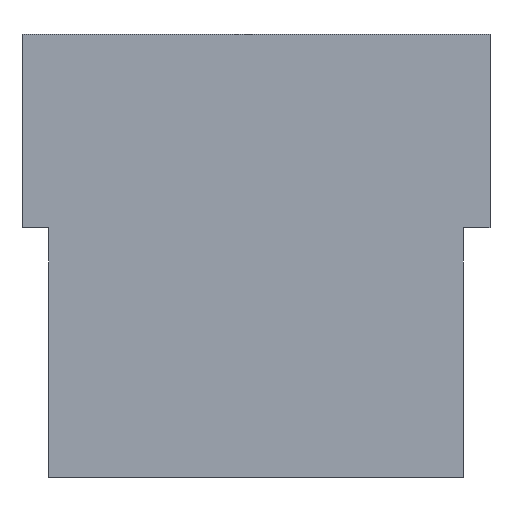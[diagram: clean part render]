
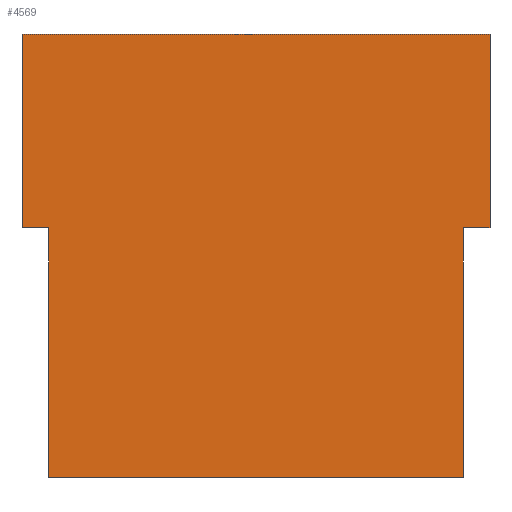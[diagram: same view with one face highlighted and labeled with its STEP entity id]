
A CAD part, front view. The second image highlights one B-rep face of the part: STEP entity #4569.
In plain terms, the highlighted planar face has unit normal (0, -1, 0).
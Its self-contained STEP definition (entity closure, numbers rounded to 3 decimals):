
#89 = VERTEX_POINT ( 'NONE', #2042 ) ;
#93 = EDGE_CURVE ( 'NONE', #89, #4918, #3731, .T. ) ;
#120 = EDGE_CURVE ( 'NONE', #4918, #233, #3376, .T. ) ;
#163 = LINE ( 'NONE', #4018, #1761 ) ;
#189 = CARTESIAN_POINT ( 'NONE',  ( 6.65, -3.15, -7.1 ) ) ;
#223 = DIRECTION ( 'NONE',  ( 0., 1., 0. ) ) ;
#233 = VERTEX_POINT ( 'NONE', #2596 ) ;
#333 = ORIENTED_EDGE ( 'NONE', *, *, #1063, .F. ) ;
#367 = VECTOR ( 'NONE', #423, 1000. ) ;
#370 = CARTESIAN_POINT ( 'NONE',  ( 7.5, -3.15, 0.9 ) ) ;
#423 = DIRECTION ( 'NONE',  ( 1., 0., 0. ) ) ;
#575 = VECTOR ( 'NONE', #2859, 1000. ) ;
#775 = PLANE ( 'NONE',  #2057 ) ;
#853 = ORIENTED_EDGE ( 'NONE', *, *, #120, .F. ) ;
#1063 = EDGE_CURVE ( 'NONE', #4021, #5097, #4996, .T. ) ;
#1168 = CARTESIAN_POINT ( 'NONE',  ( 7.5, -3.15, 7.1 ) ) ;
#1298 = VERTEX_POINT ( 'NONE', #2502 ) ;
#1385 = CARTESIAN_POINT ( 'NONE',  ( -7.5, -3.15, 7.1 ) ) ;
#1613 = VECTOR ( 'NONE', #2483, 1000. ) ;
#1621 = CARTESIAN_POINT ( 'NONE',  ( -6.65, -3.15, 23.369 ) ) ;
#1627 = CARTESIAN_POINT ( 'NONE',  ( 7.5, -3.15, -7.1 ) ) ;
#1636 = DIRECTION ( 'NONE',  ( 0., 0., 1. ) ) ;
#1679 = LINE ( 'NONE', #370, #367 ) ;
#1685 = CARTESIAN_POINT ( 'NONE',  ( 6.65, -3.15, 23.369 ) ) ;
#1746 = CARTESIAN_POINT ( 'NONE',  ( 7.5, -3.15, 7.1 ) ) ;
#1761 = VECTOR ( 'NONE', #3554, 1000. ) ;
#1814 = CARTESIAN_POINT ( 'NONE',  ( -7.5, -3.15, 0.9 ) ) ;
#1950 = ORIENTED_EDGE ( 'NONE', *, *, #93, .F. ) ;
#2017 = EDGE_CURVE ( 'NONE', #1298, #233, #5423, .T. ) ;
#2042 = CARTESIAN_POINT ( 'NONE',  ( 6.65, -3.15, 0.9 ) ) ;
#2057 = AXIS2_PLACEMENT_3D ( 'NONE', #5282, #223, #1636 ) ;
#2076 = CARTESIAN_POINT ( 'NONE',  ( 7.5, -3.15, 0.9 ) ) ;
#2279 = DIRECTION ( 'NONE',  ( 1., 0., 0. ) ) ;
#2339 = FACE_OUTER_BOUND ( 'NONE', #5420, .T. ) ;
#2483 = DIRECTION ( 'NONE',  ( 0., 0., -1. ) ) ;
#2502 = CARTESIAN_POINT ( 'NONE',  ( -6.65, -3.15, 0.9 ) ) ;
#2596 = CARTESIAN_POINT ( 'NONE',  ( -6.65, -3.15, -7.1 ) ) ;
#2859 = DIRECTION ( 'NONE',  ( 0., 0., -1. ) ) ;
#3008 = DIRECTION ( 'NONE',  ( 0., 0., -1. ) ) ;
#3053 = DIRECTION ( 'NONE',  ( 0., 0., -1. ) ) ;
#3288 = VECTOR ( 'NONE', #2279, 1000. ) ;
#3376 = LINE ( 'NONE', #1627, #5424 ) ;
#3436 = LINE ( 'NONE', #1385, #3923 ) ;
#3554 = DIRECTION ( 'NONE',  ( -1., 0., 0. ) ) ;
#3561 = EDGE_CURVE ( 'NONE', #3642, #1298, #4780, .T. ) ;
#3618 = VECTOR ( 'NONE', #3008, 1000. ) ;
#3642 = VERTEX_POINT ( 'NONE', #1814 ) ;
#3731 = LINE ( 'NONE', #1685, #1613 ) ;
#3801 = ORIENTED_EDGE ( 'NONE', *, *, #2017, .T. ) ;
#3825 = CARTESIAN_POINT ( 'NONE',  ( -7.5, -3.15, 7.1 ) ) ;
#3863 = VERTEX_POINT ( 'NONE', #3825 ) ;
#3923 = VECTOR ( 'NONE', #3053, 1000. ) ;
#4018 = CARTESIAN_POINT ( 'NONE',  ( 7.5, -3.15, 7.1 ) ) ;
#4021 = VERTEX_POINT ( 'NONE', #1746 ) ;
#4026 = EDGE_CURVE ( 'NONE', #3863, #3642, #3436, .T. ) ;
#4047 = ORIENTED_EDGE ( 'NONE', *, *, #4308, .T. ) ;
#4307 = CARTESIAN_POINT ( 'NONE',  ( -6.65, -3.15, 0.9 ) ) ;
#4308 = EDGE_CURVE ( 'NONE', #89, #5097, #1679, .T. ) ;
#4376 = ORIENTED_EDGE ( 'NONE', *, *, #4900, .T. ) ;
#4569 = ADVANCED_FACE ( 'NONE', ( #2339 ), #775, .F. ) ;
#4780 = LINE ( 'NONE', #4307, #3288 ) ;
#4900 = EDGE_CURVE ( 'NONE', #4021, #3863, #163, .T. ) ;
#4918 = VERTEX_POINT ( 'NONE', #189 ) ;
#4996 = LINE ( 'NONE', #1168, #575 ) ;
#5009 = DIRECTION ( 'NONE',  ( -1., 0., 0. ) ) ;
#5097 = VERTEX_POINT ( 'NONE', #2076 ) ;
#5128 = ORIENTED_EDGE ( 'NONE', *, *, #3561, .T. ) ;
#5165 = ORIENTED_EDGE ( 'NONE', *, *, #4026, .T. ) ;
#5282 = CARTESIAN_POINT ( 'NONE',  ( 7.5, -3.15, 7.1 ) ) ;
#5420 = EDGE_LOOP ( 'NONE', ( #853, #1950, #4047, #333, #4376, #5165, #5128, #3801 ) ) ;
#5423 = LINE ( 'NONE', #1621, #3618 ) ;
#5424 = VECTOR ( 'NONE', #5009, 1000. ) ;
